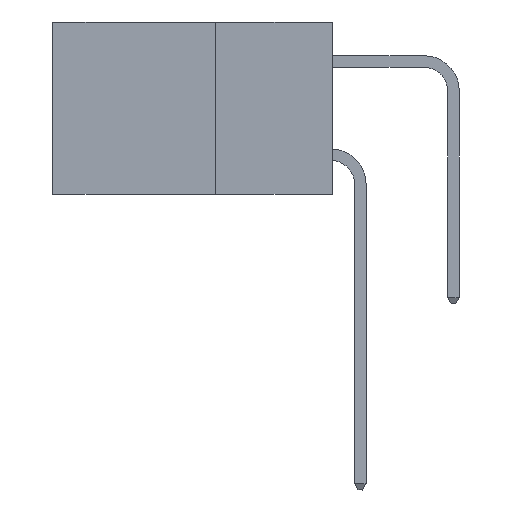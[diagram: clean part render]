
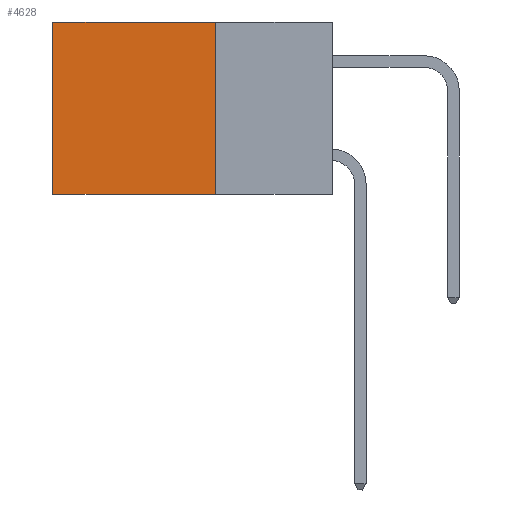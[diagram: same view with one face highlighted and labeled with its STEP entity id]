
A CAD part, left-side view. The second image highlights one B-rep face of the part: STEP entity #4628.
In plain terms, the highlighted planar face has unit normal (-1, 0, 0).
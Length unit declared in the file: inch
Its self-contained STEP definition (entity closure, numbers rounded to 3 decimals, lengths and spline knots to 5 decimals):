
#382 = CARTESIAN_POINT ( 'NONE',  ( 0.2615, 0.25, -0.37 ) ) ;
#1876 = LINE ( 'NONE', #7837, #4514 ) ;
#1903 = VECTOR ( 'NONE', #5533, 39.37008 ) ;
#2147 = LINE ( 'NONE', #11372, #1903 ) ;
#2348 = VERTEX_POINT ( 'NONE', #8741 ) ;
#2470 = EDGE_LOOP ( 'NONE', ( #3371, #12424, #4082, #4083 ) ) ;
#2788 = VERTEX_POINT ( 'NONE', #11926 ) ;
#2792 = DIRECTION ( 'NONE',  ( 1., 0., 0. ) ) ;
#3371 = ORIENTED_EDGE ( 'NONE', *, *, #7902, .T. ) ;
#3742 = VERTEX_POINT ( 'NONE', #7314 ) ;
#4082 = ORIENTED_EDGE ( 'NONE', *, *, #13767, .F. ) ;
#4083 = ORIENTED_EDGE ( 'NONE', *, *, #9314, .T. ) ;
#4279 = DIRECTION ( 'NONE',  ( 0., 1., 0. ) ) ;
#4514 = VECTOR ( 'NONE', #4279, 39.37008 ) ;
#4628 = ADVANCED_FACE ( 'NONE', ( #13252 ), #6123, .F. ) ;
#4914 = DIRECTION ( 'NONE',  ( 0., 1., 0. ) ) ;
#5480 = CARTESIAN_POINT ( 'NONE',  ( 0.2615, 0.6, -0.37 ) ) ;
#5533 = DIRECTION ( 'NONE',  ( 0., 0., -1. ) ) ;
#5657 = DIRECTION ( 'NONE',  ( 0., 0., -1. ) ) ;
#6123 = PLANE ( 'NONE',  #13321 ) ;
#7096 = CARTESIAN_POINT ( 'NONE',  ( 0.2615, 0.25, 0. ) ) ;
#7314 = CARTESIAN_POINT ( 'NONE',  ( 0.2615, 0.25, 0. ) ) ;
#7837 = CARTESIAN_POINT ( 'NONE',  ( 0.2615, 0.25, -0.37 ) ) ;
#7902 = EDGE_CURVE ( 'NONE', #2348, #10051, #12423, .T. ) ;
#8004 = VECTOR ( 'NONE', #4914, 39.37008 ) ;
#8473 = LINE ( 'NONE', #7096, #8004 ) ;
#8701 = DIRECTION ( 'NONE',  ( 0., 0., -1. ) ) ;
#8741 = CARTESIAN_POINT ( 'NONE',  ( 0.2615, 0.6, 0. ) ) ;
#8853 = CARTESIAN_POINT ( 'NONE',  ( 0.2615, 0.6, -0.37 ) ) ;
#9314 = EDGE_CURVE ( 'NONE', #3742, #2348, #8473, .T. ) ;
#10051 = VERTEX_POINT ( 'NONE', #5480 ) ;
#11372 = CARTESIAN_POINT ( 'NONE',  ( 0.2615, 0.25, -0.37 ) ) ;
#11739 = VECTOR ( 'NONE', #5657, 39.37008 ) ;
#11926 = CARTESIAN_POINT ( 'NONE',  ( 0.2615, 0.25, -0.37 ) ) ;
#12423 = LINE ( 'NONE', #8853, #11739 ) ;
#12424 = ORIENTED_EDGE ( 'NONE', *, *, #12674, .F. ) ;
#12674 = EDGE_CURVE ( 'NONE', #2788, #10051, #1876, .T. ) ;
#13252 = FACE_OUTER_BOUND ( 'NONE', #2470, .T. ) ;
#13321 = AXIS2_PLACEMENT_3D ( 'NONE', #382, #2792, #8701 ) ;
#13767 = EDGE_CURVE ( 'NONE', #3742, #2788, #2147, .T. ) ;
